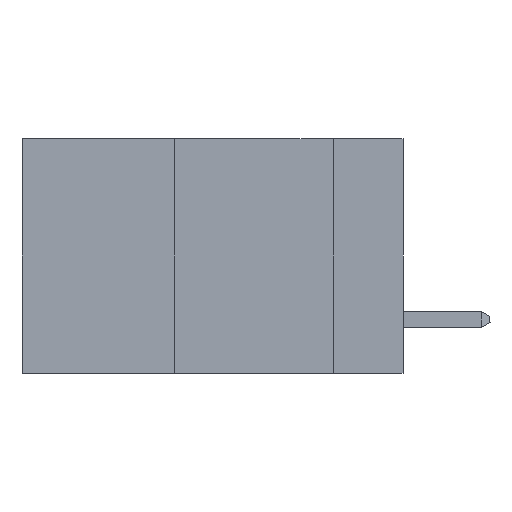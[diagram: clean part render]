
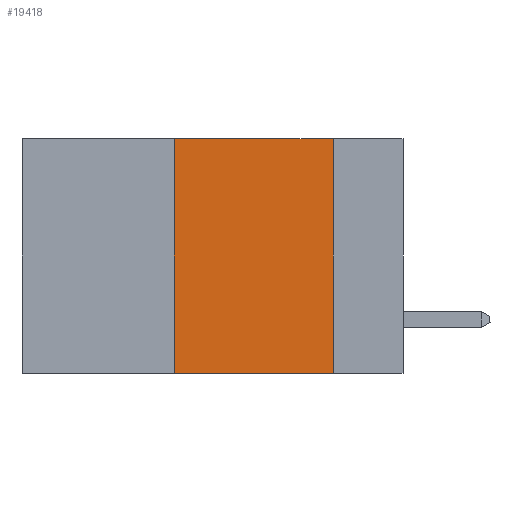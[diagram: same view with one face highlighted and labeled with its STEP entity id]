
A CAD part, left-side view. The second image highlights one B-rep face of the part: STEP entity #19418.
In plain terms, the highlighted planar face has unit normal (-1, 0, 0).
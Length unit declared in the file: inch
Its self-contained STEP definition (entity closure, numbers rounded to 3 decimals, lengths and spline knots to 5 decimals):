
#501 = EDGE_CURVE ( 'NONE', #20286, #22736, #14757, .T. ) ;
#1316 = DIRECTION ( 'NONE',  ( 0., -1., 0. ) ) ;
#2881 = CARTESIAN_POINT ( 'NONE',  ( 0., 0.36, 0. ) ) ;
#3894 = DIRECTION ( 'NONE',  ( 1., 0., 0. ) ) ;
#4072 = LINE ( 'NONE', #9502, #18284 ) ;
#5118 = LINE ( 'NONE', #2881, #7748 ) ;
#5446 = CARTESIAN_POINT ( 'NONE',  ( 0., 0.11, 0. ) ) ;
#7748 = VECTOR ( 'NONE', #24119, 39.37008 ) ;
#7867 = ORIENTED_EDGE ( 'NONE', *, *, #501, .T. ) ;
#8414 = ORIENTED_EDGE ( 'NONE', *, *, #26538, .F. ) ;
#9272 = CARTESIAN_POINT ( 'NONE',  ( 0., 0.6, -0.37 ) ) ;
#9502 = CARTESIAN_POINT ( 'NONE',  ( 0., 0.11, 0. ) ) ;
#10543 = VERTEX_POINT ( 'NONE', #5446 ) ;
#10705 = CARTESIAN_POINT ( 'NONE',  ( 0., 0.36, 0. ) ) ;
#11420 = DIRECTION ( 'NONE',  ( 0., -1., 0. ) ) ;
#11539 = DIRECTION ( 'NONE',  ( 0., 0., -1. ) ) ;
#11708 = AXIS2_PLACEMENT_3D ( 'NONE', #18766, #3894, #24777 ) ;
#12171 = EDGE_LOOP ( 'NONE', ( #19535, #22222, #8414, #7867 ) ) ;
#13951 = CARTESIAN_POINT ( 'NONE',  ( 0., 0.6, 0. ) ) ;
#14061 = EDGE_CURVE ( 'NONE', #17286, #10543, #23192, .T. ) ;
#14175 = CARTESIAN_POINT ( 'NONE',  ( 0., 0.36, -0.37 ) ) ;
#14428 = VECTOR ( 'NONE', #11420, 39.37008 ) ;
#14757 = LINE ( 'NONE', #9272, #14428 ) ;
#15978 = VECTOR ( 'NONE', #1316, 39.37008 ) ;
#16812 = CARTESIAN_POINT ( 'NONE',  ( 0., 0.11, -0.37 ) ) ;
#17286 = VERTEX_POINT ( 'NONE', #10705 ) ;
#18284 = VECTOR ( 'NONE', #11539, 39.37008 ) ;
#18766 = CARTESIAN_POINT ( 'NONE',  ( 0., 0.6, 0. ) ) ;
#19418 = ADVANCED_FACE ( 'NONE', ( #26946 ), #26452, .F. ) ;
#19535 = ORIENTED_EDGE ( 'NONE', *, *, #27245, .F. ) ;
#20286 = VERTEX_POINT ( 'NONE', #14175 ) ;
#22222 = ORIENTED_EDGE ( 'NONE', *, *, #14061, .F. ) ;
#22736 = VERTEX_POINT ( 'NONE', #16812 ) ;
#23192 = LINE ( 'NONE', #13951, #15978 ) ;
#24119 = DIRECTION ( 'NONE',  ( 0., 0., 1. ) ) ;
#24777 = DIRECTION ( 'NONE',  ( 0., 0., -1. ) ) ;
#26452 = PLANE ( 'NONE',  #11708 ) ;
#26538 = EDGE_CURVE ( 'NONE', #20286, #17286, #5118, .T. ) ;
#26946 = FACE_OUTER_BOUND ( 'NONE', #12171, .T. ) ;
#27245 = EDGE_CURVE ( 'NONE', #10543, #22736, #4072, .T. ) ;
